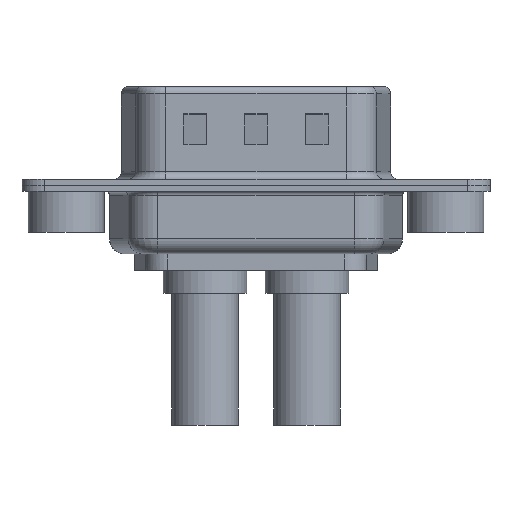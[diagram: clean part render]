
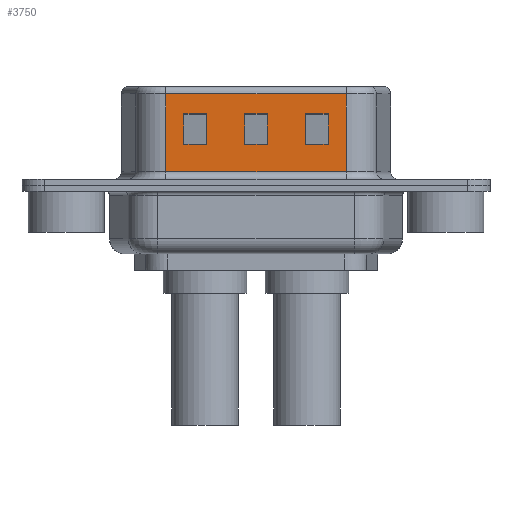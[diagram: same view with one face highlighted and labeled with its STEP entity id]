
A CAD part, front view. The second image highlights one B-rep face of the part: STEP entity #3750.
In plain terms, the highlighted planar face has unit normal (0, -1, 0).
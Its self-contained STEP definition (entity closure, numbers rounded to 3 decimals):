
#66 = VERTEX_POINT ( 'NONE', #3537 ) ;
#144 = CARTESIAN_POINT ( 'NONE',  ( 17.25, -4.58, 4.705 ) ) ;
#198 = VECTOR ( 'NONE', #10922, 1000. ) ;
#528 = LINE ( 'NONE', #1797, #9223 ) ;
#544 = CARTESIAN_POINT ( 'NONE',  ( 9.25, -4.58, 2.705 ) ) ;
#612 = VERTEX_POINT ( 'NONE', #2172 ) ;
#713 = CARTESIAN_POINT ( 'NONE',  ( 6.55, -4.58, 6.52 ) ) ;
#805 = VECTOR ( 'NONE', #4696, 1000. ) ;
#866 = AXIS2_PLACEMENT_3D ( 'NONE', #5604, #12943, #1656 ) ;
#893 = CARTESIAN_POINT ( 'NONE',  ( 14.45, -4.58, 4.705 ) ) ;
#932 = VERTEX_POINT ( 'NONE', #12730 ) ;
#1264 = LINE ( 'NONE', #6334, #9572 ) ;
#1273 = PLANE ( 'NONE',  #866 ) ;
#1277 = CARTESIAN_POINT ( 'NONE',  ( 15.75, -4.58, 4.705 ) ) ;
#1307 = EDGE_CURVE ( 'NONE', #66, #8231, #12224, .T. ) ;
#1501 = EDGE_CURVE ( 'NONE', #6685, #5527, #12387, .T. ) ;
#1656 = DIRECTION ( 'NONE',  ( 0., 0., 1. ) ) ;
#1693 = VERTEX_POINT ( 'NONE', #3077 ) ;
#1797 = CARTESIAN_POINT ( 'NONE',  ( 18.45, -4.58, 6.02 ) ) ;
#1937 = EDGE_LOOP ( 'NONE', ( #7698, #13975, #11897, #4060 ) ) ;
#1955 = EDGE_CURVE ( 'NONE', #8582, #6685, #3631, .T. ) ;
#2119 = CARTESIAN_POINT ( 'NONE',  ( 11.75, -4.58, 6.52 ) ) ;
#2138 = DIRECTION ( 'NONE',  ( -1., 0., 0. ) ) ;
#2172 = CARTESIAN_POINT ( 'NONE',  ( 11.75, -4.58, 4.705 ) ) ;
#2209 = EDGE_CURVE ( 'NONE', #612, #932, #4147, .T. ) ;
#2234 = VECTOR ( 'NONE', #14546, 1000. ) ;
#2534 = DIRECTION ( 'NONE',  ( 0., 0., -1. ) ) ;
#2857 = FACE_BOUND ( 'NONE', #13888, .T. ) ;
#2915 = VECTOR ( 'NONE', #13389, 1000. ) ;
#2952 = CARTESIAN_POINT ( 'NONE',  ( 14.45, -4.58, 2.705 ) ) ;
#2985 = ORIENTED_EDGE ( 'NONE', *, *, #13100, .T. ) ;
#3077 = CARTESIAN_POINT ( 'NONE',  ( 9.25, -4.58, 4.705 ) ) ;
#3130 = LINE ( 'NONE', #12849, #12083 ) ;
#3249 = CARTESIAN_POINT ( 'NONE',  ( 18.45, -4.58, 0.9 ) ) ;
#3537 = CARTESIAN_POINT ( 'NONE',  ( 18.45, -4.58, 6.02 ) ) ;
#3570 = LINE ( 'NONE', #12404, #8464 ) ;
#3621 = EDGE_CURVE ( 'NONE', #4404, #9630, #4634, .T. ) ;
#3631 = LINE ( 'NONE', #11059, #198 ) ;
#3726 = CARTESIAN_POINT ( 'NONE',  ( 11.75, -4.58, 2.705 ) ) ;
#3750 = ADVANCED_FACE ( 'NONE', ( #8847, #2857, #11826, #14499 ), #1273, .F. ) ;
#3831 = LINE ( 'NONE', #2952, #9445 ) ;
#3942 = DIRECTION ( 'NONE',  ( 1., 0., 0. ) ) ;
#3953 = ORIENTED_EDGE ( 'NONE', *, *, #1307, .F. ) ;
#4060 = ORIENTED_EDGE ( 'NONE', *, *, #8335, .T. ) ;
#4126 = ORIENTED_EDGE ( 'NONE', *, *, #4212, .T. ) ;
#4147 = LINE ( 'NONE', #11939, #9779 ) ;
#4205 = CARTESIAN_POINT ( 'NONE',  ( 6.55, -4.58, 0.9 ) ) ;
#4212 = EDGE_CURVE ( 'NONE', #9630, #8231, #7954, .T. ) ;
#4249 = ORIENTED_EDGE ( 'NONE', *, *, #7505, .T. ) ;
#4321 = EDGE_CURVE ( 'NONE', #8064, #9294, #9203, .T. ) ;
#4404 = VERTEX_POINT ( 'NONE', #6369 ) ;
#4634 = LINE ( 'NONE', #713, #13251 ) ;
#4696 = DIRECTION ( 'NONE',  ( 0., 0., 1. ) ) ;
#4896 = EDGE_CURVE ( 'NONE', #1693, #12997, #3570, .T. ) ;
#4948 = CARTESIAN_POINT ( 'NONE',  ( 7.75, -4.58, 4.705 ) ) ;
#5202 = ORIENTED_EDGE ( 'NONE', *, *, #9730, .T. ) ;
#5359 = ORIENTED_EDGE ( 'NONE', *, *, #7985, .T. ) ;
#5432 = VECTOR ( 'NONE', #10040, 1000. ) ;
#5527 = VERTEX_POINT ( 'NONE', #12670 ) ;
#5604 = CARTESIAN_POINT ( 'NONE',  ( 18.45, -4.58, 6.52 ) ) ;
#5821 = VERTEX_POINT ( 'NONE', #14558 ) ;
#5926 = DIRECTION ( 'NONE',  ( -1., 0., 0. ) ) ;
#6213 = VECTOR ( 'NONE', #2138, 1000. ) ;
#6334 = CARTESIAN_POINT ( 'NONE',  ( 13.25, -4.58, 6.52 ) ) ;
#6369 = CARTESIAN_POINT ( 'NONE',  ( 6.55, -4.58, 6.02 ) ) ;
#6371 = CARTESIAN_POINT ( 'NONE',  ( 13.25, -4.58, 2.705 ) ) ;
#6682 = CARTESIAN_POINT ( 'NONE',  ( 22.45, -4.58, 2.705 ) ) ;
#6685 = VERTEX_POINT ( 'NONE', #144 ) ;
#7505 = EDGE_CURVE ( 'NONE', #10012, #8582, #3130, .T. ) ;
#7513 = VECTOR ( 'NONE', #8808, 1000. ) ;
#7666 = ORIENTED_EDGE ( 'NONE', *, *, #1501, .T. ) ;
#7698 = ORIENTED_EDGE ( 'NONE', *, *, #2209, .T. ) ;
#7954 = LINE ( 'NONE', #3249, #10609 ) ;
#7985 = EDGE_CURVE ( 'NONE', #12997, #5821, #3831, .T. ) ;
#8064 = VERTEX_POINT ( 'NONE', #6371 ) ;
#8153 = ORIENTED_EDGE ( 'NONE', *, *, #9250, .T. ) ;
#8225 = LINE ( 'NONE', #6682, #2234 ) ;
#8231 = VERTEX_POINT ( 'NONE', #13168 ) ;
#8335 = EDGE_CURVE ( 'NONE', #9294, #612, #11407, .T. ) ;
#8464 = VECTOR ( 'NONE', #2534, 1000. ) ;
#8582 = VERTEX_POINT ( 'NONE', #1277 ) ;
#8619 = DIRECTION ( 'NONE',  ( -1., 0., 0. ) ) ;
#8697 = CARTESIAN_POINT ( 'NONE',  ( 18.45, -4.58, 6.52 ) ) ;
#8808 = DIRECTION ( 'NONE',  ( 1., 0., 0. ) ) ;
#8847 = FACE_BOUND ( 'NONE', #11733, .T. ) ;
#9088 = EDGE_CURVE ( 'NONE', #5527, #10012, #8225, .T. ) ;
#9203 = LINE ( 'NONE', #14377, #6213 ) ;
#9223 = VECTOR ( 'NONE', #8619, 1000. ) ;
#9250 = EDGE_CURVE ( 'NONE', #5821, #14004, #12424, .T. ) ;
#9294 = VERTEX_POINT ( 'NONE', #3726 ) ;
#9445 = VECTOR ( 'NONE', #5926, 1000. ) ;
#9572 = VECTOR ( 'NONE', #14189, 1000. ) ;
#9621 = DIRECTION ( 'NONE',  ( 0., 0., 1. ) ) ;
#9630 = VERTEX_POINT ( 'NONE', #4205 ) ;
#9730 = EDGE_CURVE ( 'NONE', #14004, #1693, #10528, .T. ) ;
#9779 = VECTOR ( 'NONE', #3942, 1000. ) ;
#9924 = ORIENTED_EDGE ( 'NONE', *, *, #3621, .T. ) ;
#10012 = VERTEX_POINT ( 'NONE', #11639 ) ;
#10040 = DIRECTION ( 'NONE',  ( 0., 0., 1. ) ) ;
#10148 = VECTOR ( 'NONE', #13433, 1000. ) ;
#10528 = LINE ( 'NONE', #893, #7513 ) ;
#10609 = VECTOR ( 'NONE', #13933, 1000. ) ;
#10922 = DIRECTION ( 'NONE',  ( 1., 0., 0. ) ) ;
#11059 = CARTESIAN_POINT ( 'NONE',  ( 22.45, -4.58, 4.705 ) ) ;
#11287 = CARTESIAN_POINT ( 'NONE',  ( 17.25, -4.58, 6.52 ) ) ;
#11407 = LINE ( 'NONE', #2119, #5432 ) ;
#11546 = ORIENTED_EDGE ( 'NONE', *, *, #9088, .T. ) ;
#11639 = CARTESIAN_POINT ( 'NONE',  ( 15.75, -4.58, 2.705 ) ) ;
#11733 = EDGE_LOOP ( 'NONE', ( #12636, #5359, #8153, #5202 ) ) ;
#11826 = FACE_BOUND ( 'NONE', #1937, .T. ) ;
#11897 = ORIENTED_EDGE ( 'NONE', *, *, #4321, .T. ) ;
#11939 = CARTESIAN_POINT ( 'NONE',  ( 18.45, -4.58, 4.705 ) ) ;
#12083 = VECTOR ( 'NONE', #9621, 1000. ) ;
#12224 = LINE ( 'NONE', #8697, #2915 ) ;
#12297 = DIRECTION ( 'NONE',  ( 0., 0., -1. ) ) ;
#12387 = LINE ( 'NONE', #11287, #10148 ) ;
#12404 = CARTESIAN_POINT ( 'NONE',  ( 9.25, -4.58, 6.52 ) ) ;
#12424 = LINE ( 'NONE', #14691, #805 ) ;
#12636 = ORIENTED_EDGE ( 'NONE', *, *, #4896, .T. ) ;
#12670 = CARTESIAN_POINT ( 'NONE',  ( 17.25, -4.58, 2.705 ) ) ;
#12730 = CARTESIAN_POINT ( 'NONE',  ( 13.25, -4.58, 4.705 ) ) ;
#12849 = CARTESIAN_POINT ( 'NONE',  ( 15.75, -4.58, 6.52 ) ) ;
#12943 = DIRECTION ( 'NONE',  ( 0., 1., 0. ) ) ;
#12997 = VERTEX_POINT ( 'NONE', #544 ) ;
#13064 = EDGE_CURVE ( 'NONE', #932, #8064, #1264, .T. ) ;
#13100 = EDGE_CURVE ( 'NONE', #66, #4404, #528, .T. ) ;
#13168 = CARTESIAN_POINT ( 'NONE',  ( 18.45, -4.58, 0.9 ) ) ;
#13251 = VECTOR ( 'NONE', #12297, 1000. ) ;
#13326 = EDGE_LOOP ( 'NONE', ( #3953, #2985, #9924, #4126 ) ) ;
#13389 = DIRECTION ( 'NONE',  ( 0., 0., -1. ) ) ;
#13433 = DIRECTION ( 'NONE',  ( 0., 0., -1. ) ) ;
#13879 = ORIENTED_EDGE ( 'NONE', *, *, #1955, .T. ) ;
#13888 = EDGE_LOOP ( 'NONE', ( #7666, #11546, #4249, #13879 ) ) ;
#13933 = DIRECTION ( 'NONE',  ( 1., 0., 0. ) ) ;
#13975 = ORIENTED_EDGE ( 'NONE', *, *, #13064, .T. ) ;
#14004 = VERTEX_POINT ( 'NONE', #4948 ) ;
#14189 = DIRECTION ( 'NONE',  ( 0., 0., -1. ) ) ;
#14377 = CARTESIAN_POINT ( 'NONE',  ( 18.45, -4.58, 2.705 ) ) ;
#14499 = FACE_OUTER_BOUND ( 'NONE', #13326, .T. ) ;
#14546 = DIRECTION ( 'NONE',  ( -1., 0., 0. ) ) ;
#14558 = CARTESIAN_POINT ( 'NONE',  ( 7.75, -4.58, 2.705 ) ) ;
#14691 = CARTESIAN_POINT ( 'NONE',  ( 7.75, -4.58, 6.52 ) ) ;
